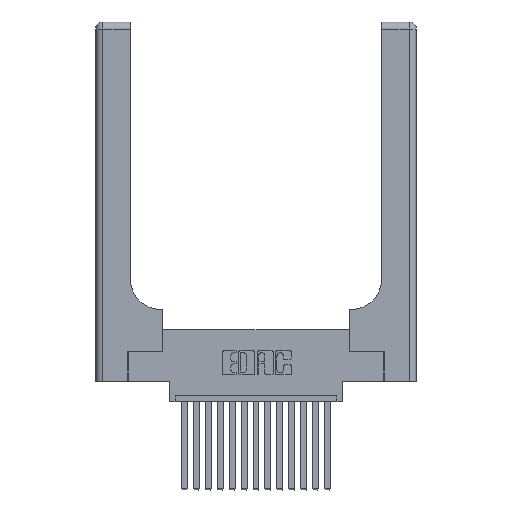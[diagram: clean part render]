
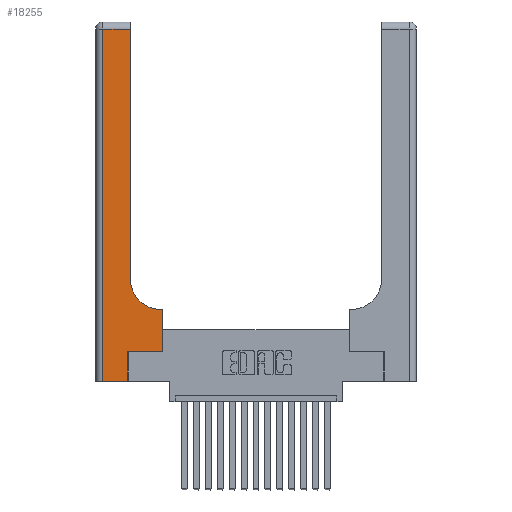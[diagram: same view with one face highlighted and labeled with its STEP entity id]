
A CAD part, top view. The second image highlights one B-rep face of the part: STEP entity #18255.
In plain terms, the highlighted planar face has unit normal (0, 0, 1).
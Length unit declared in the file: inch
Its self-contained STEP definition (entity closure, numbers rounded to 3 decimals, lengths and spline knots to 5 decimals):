
#825 = VECTOR ( 'NONE', #12643, 39.37008 ) ;
#1119 = CARTESIAN_POINT ( 'NONE',  ( 0., 2.94, 0.37 ) ) ;
#1344 = CARTESIAN_POINT ( 'NONE',  ( 0.269, 0.25, 0.37 ) ) ;
#1375 = DIRECTION ( 'NONE',  ( 0., 1., 0. ) ) ;
#1633 = VECTOR ( 'NONE', #14600, 39.37008 ) ;
#1689 = ORIENTED_EDGE ( 'NONE', *, *, #15321, .T. ) ;
#1812 = CARTESIAN_POINT ( 'NONE',  ( 0.2915, 2.94, 0.37 ) ) ;
#2125 = CARTESIAN_POINT ( 'NONE',  ( 0.269, 0., 0.37 ) ) ;
#2378 = CARTESIAN_POINT ( 'NONE',  ( 0.06, 2.94, 0.37 ) ) ;
#3138 = VERTEX_POINT ( 'NONE', #9741 ) ;
#3161 = CARTESIAN_POINT ( 'NONE',  ( 0.5585, 0.6, 0.37 ) ) ;
#3257 = VERTEX_POINT ( 'NONE', #1344 ) ;
#3446 = EDGE_LOOP ( 'NONE', ( #5591, #18043, #5619, #1689, #18837, #17843, #4489, #11865, #6034 ) ) ;
#3584 = VERTEX_POINT ( 'NONE', #13996 ) ;
#4260 = DIRECTION ( 'NONE',  ( -1., 0., 0. ) ) ;
#4489 = ORIENTED_EDGE ( 'NONE', *, *, #12360, .T. ) ;
#4792 = DIRECTION ( 'NONE',  ( 0., 1., 0. ) ) ;
#4990 = CARTESIAN_POINT ( 'NONE',  ( 0., 0., 0.37 ) ) ;
#5181 = AXIS2_PLACEMENT_3D ( 'NONE', #9074, #16093, #7545 ) ;
#5515 = LINE ( 'NONE', #5964, #1633 ) ;
#5591 = ORIENTED_EDGE ( 'NONE', *, *, #9752, .T. ) ;
#5619 = ORIENTED_EDGE ( 'NONE', *, *, #5623, .T. ) ;
#5623 = EDGE_CURVE ( 'NONE', #18711, #3584, #18771, .T. ) ;
#5644 = DIRECTION ( 'NONE',  ( 0., 0., -1. ) ) ;
#5661 = VERTEX_POINT ( 'NONE', #3161 ) ;
#5683 = VERTEX_POINT ( 'NONE', #1812 ) ;
#5719 = CIRCLE ( 'NONE', #5181, 0.25 ) ;
#5843 = VECTOR ( 'NONE', #7783, 39.37008 ) ;
#5964 = CARTESIAN_POINT ( 'NONE',  ( 0.269, 0.25, 0.37 ) ) ;
#6009 = DIRECTION ( 'NONE',  ( 0., -1., 0. ) ) ;
#6034 = ORIENTED_EDGE ( 'NONE', *, *, #18402, .T. ) ;
#7179 = VECTOR ( 'NONE', #6009, 39.37008 ) ;
#7462 = CARTESIAN_POINT ( 'NONE',  ( 0.06, 3., 0.37 ) ) ;
#7545 = DIRECTION ( 'NONE',  ( 1., 0., 0. ) ) ;
#7626 = EDGE_CURVE ( 'NONE', #3257, #7707, #5515, .T. ) ;
#7659 = LINE ( 'NONE', #1119, #825 ) ;
#7707 = VERTEX_POINT ( 'NONE', #14153 ) ;
#7783 = DIRECTION ( 'NONE',  ( 1., 0., 0. ) ) ;
#8277 = EDGE_CURVE ( 'NONE', #5661, #11882, #13466, .T. ) ;
#8449 = CARTESIAN_POINT ( 'NONE',  ( 0.2915, 3., 0.37 ) ) ;
#8504 = PLANE ( 'NONE',  #12724 ) ;
#8638 = VECTOR ( 'NONE', #4792, 39.37008 ) ;
#9074 = CARTESIAN_POINT ( 'NONE',  ( 0.5415, 0.85, 0.37 ) ) ;
#9079 = VECTOR ( 'NONE', #1375, 39.37008 ) ;
#9145 = CARTESIAN_POINT ( 'NONE',  ( 0.2915, 0.6, 0.37 ) ) ;
#9352 = FACE_OUTER_BOUND ( 'NONE', #3446, .T. ) ;
#9741 = CARTESIAN_POINT ( 'NONE',  ( 0.2915, 0.85, 0.37 ) ) ;
#9752 = EDGE_CURVE ( 'NONE', #3138, #5683, #12932, .T. ) ;
#9972 = CARTESIAN_POINT ( 'NONE',  ( 0., 3., 0.37 ) ) ;
#10044 = DIRECTION ( 'NONE',  ( -1., 0., 0. ) ) ;
#10528 = VECTOR ( 'NONE', #10044, 39.37008 ) ;
#11057 = VERTEX_POINT ( 'NONE', #13361 ) ;
#11865 = ORIENTED_EDGE ( 'NONE', *, *, #8277, .T. ) ;
#11882 = VERTEX_POINT ( 'NONE', #13689 ) ;
#12360 = EDGE_CURVE ( 'NONE', #7707, #5661, #18012, .T. ) ;
#12643 = DIRECTION ( 'NONE',  ( -1., 0., 0. ) ) ;
#12724 = AXIS2_PLACEMENT_3D ( 'NONE', #9972, #5644, #4260 ) ;
#12932 = LINE ( 'NONE', #8449, #9079 ) ;
#13361 = CARTESIAN_POINT ( 'NONE',  ( 0.269, 0., 0.37 ) ) ;
#13466 = LINE ( 'NONE', #9145, #10528 ) ;
#13501 = VECTOR ( 'NONE', #18075, 39.37008 ) ;
#13689 = CARTESIAN_POINT ( 'NONE',  ( 0.5415, 0.6, 0.37 ) ) ;
#13996 = CARTESIAN_POINT ( 'NONE',  ( 0.06, 0., 0.37 ) ) ;
#14153 = CARTESIAN_POINT ( 'NONE',  ( 0.5585, 0.25, 0.37 ) ) ;
#14263 = EDGE_CURVE ( 'NONE', #5683, #18711, #7659, .T. ) ;
#14600 = DIRECTION ( 'NONE',  ( 1., 0., 0. ) ) ;
#15321 = EDGE_CURVE ( 'NONE', #3584, #11057, #16040, .T. ) ;
#15764 = LINE ( 'NONE', #2125, #13501 ) ;
#16040 = LINE ( 'NONE', #4990, #5843 ) ;
#16093 = DIRECTION ( 'NONE',  ( 0., 0., -1. ) ) ;
#16827 = EDGE_CURVE ( 'NONE', #11057, #3257, #15764, .T. ) ;
#17796 = CARTESIAN_POINT ( 'NONE',  ( 0.5585, 0.25, 0.37 ) ) ;
#17843 = ORIENTED_EDGE ( 'NONE', *, *, #7626, .T. ) ;
#18012 = LINE ( 'NONE', #17796, #8638 ) ;
#18043 = ORIENTED_EDGE ( 'NONE', *, *, #14263, .T. ) ;
#18075 = DIRECTION ( 'NONE',  ( 0., 1., 0. ) ) ;
#18255 = ADVANCED_FACE ( 'NONE', ( #9352 ), #8504, .F. ) ;
#18402 = EDGE_CURVE ( 'NONE', #11882, #3138, #5719, .T. ) ;
#18711 = VERTEX_POINT ( 'NONE', #2378 ) ;
#18771 = LINE ( 'NONE', #7462, #7179 ) ;
#18837 = ORIENTED_EDGE ( 'NONE', *, *, #16827, .T. ) ;
